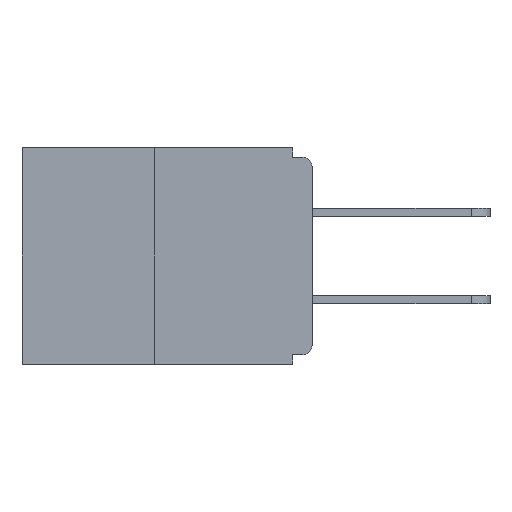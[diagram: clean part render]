
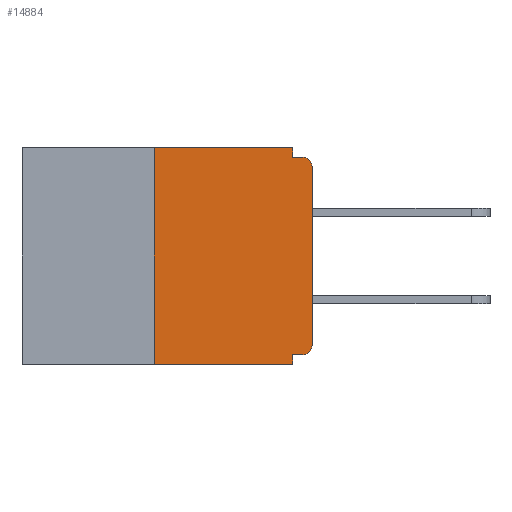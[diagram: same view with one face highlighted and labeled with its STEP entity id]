
A CAD part, left-side view. The second image highlights one B-rep face of the part: STEP entity #14884.
In plain terms, the highlighted planar face has unit normal (-1, 0, 0).
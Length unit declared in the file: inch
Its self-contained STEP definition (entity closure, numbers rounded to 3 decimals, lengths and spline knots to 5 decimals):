
#120 = ORIENTED_EDGE ( 'NONE', *, *, #15471, .T. ) ;
#579 = DIRECTION ( 'NONE',  ( 0., 0., -1. ) ) ;
#1184 = PLANE ( 'NONE',  #18767 ) ;
#1459 = CARTESIAN_POINT ( 'NONE',  ( 0., 0., 0. ) ) ;
#2770 = CARTESIAN_POINT ( 'NONE',  ( 0., 0.031, 0. ) ) ;
#2809 = VECTOR ( 'NONE', #9097, 39.37008 ) ;
#3345 = CARTESIAN_POINT ( 'NONE',  ( 0., 0.015, -0.328 ) ) ;
#3481 = VERTEX_POINT ( 'NONE', #20496 ) ;
#3826 = ORIENTED_EDGE ( 'NONE', *, *, #25433, .F. ) ;
#4639 = VERTEX_POINT ( 'NONE', #5701 ) ;
#4949 = ORIENTED_EDGE ( 'NONE', *, *, #5563, .T. ) ;
#4956 = VECTOR ( 'NONE', #579, 39.37008 ) ;
#5487 = EDGE_CURVE ( 'NONE', #21821, #3481, #13147, .T. ) ;
#5563 = EDGE_CURVE ( 'NONE', #14301, #21821, #7819, .T. ) ;
#5672 = ORIENTED_EDGE ( 'NONE', *, *, #7404, .F. ) ;
#5701 = CARTESIAN_POINT ( 'NONE',  ( 0., 0.031, 0. ) ) ;
#5748 = ORIENTED_EDGE ( 'NONE', *, *, #7896, .F. ) ;
#5768 = CARTESIAN_POINT ( 'NONE',  ( 0., 0.031, -0.328 ) ) ;
#5869 = VECTOR ( 'NONE', #22485, 39.37008 ) ;
#6130 = CARTESIAN_POINT ( 'NONE',  ( 0., 0., -0.328 ) ) ;
#6212 = AXIS2_PLACEMENT_3D ( 'NONE', #11804, #11997, #25696 ) ;
#6424 = EDGE_LOOP ( 'NONE', ( #20912, #5748, #14328, #3826, #5672, #4949, #8982, #120, #22084, #16648 ) ) ;
#6955 = AXIS2_PLACEMENT_3D ( 'NONE', #14535, #23785, #23608 ) ;
#7404 = EDGE_CURVE ( 'NONE', #14301, #9395, #20503, .T. ) ;
#7657 = CARTESIAN_POINT ( 'NONE',  ( 0., 0., -0.313 ) ) ;
#7669 = CIRCLE ( 'NONE', #6955, 0.015 ) ;
#7819 = CIRCLE ( 'NONE', #6212, 0.015 ) ;
#7896 = EDGE_CURVE ( 'NONE', #15224, #15062, #24730, .T. ) ;
#8139 = DIRECTION ( 'NONE',  ( 1., 0., 0. ) ) ;
#8410 = DIRECTION ( 'NONE',  ( 0., 1., 0. ) ) ;
#8478 = DIRECTION ( 'NONE',  ( 0., -1., 0. ) ) ;
#8982 = ORIENTED_EDGE ( 'NONE', *, *, #5487, .T. ) ;
#9097 = DIRECTION ( 'NONE',  ( 0., -1., 0. ) ) ;
#9395 = VERTEX_POINT ( 'NONE', #5768 ) ;
#9568 = LINE ( 'NONE', #15973, #2809 ) ;
#11019 = LINE ( 'NONE', #2770, #4956 ) ;
#11477 = CARTESIAN_POINT ( 'NONE',  ( 0., 0.031, -0.343 ) ) ;
#11804 = CARTESIAN_POINT ( 'NONE',  ( 0., 0.015, -0.313 ) ) ;
#11997 = DIRECTION ( 'NONE',  ( -1., 0., 0. ) ) ;
#12405 = CARTESIAN_POINT ( 'NONE',  ( 0., 0.015, -0.015 ) ) ;
#12442 = CARTESIAN_POINT ( 'NONE',  ( 0., 0.46, 0. ) ) ;
#12446 = EDGE_CURVE ( 'NONE', #4639, #26085, #11019, .T. ) ;
#13147 = LINE ( 'NONE', #1459, #27372 ) ;
#13225 = CARTESIAN_POINT ( 'NONE',  ( 0., 0.031, -0.343 ) ) ;
#13729 = VECTOR ( 'NONE', #8410, 39.37008 ) ;
#14010 = VECTOR ( 'NONE', #26837, 39.37008 ) ;
#14301 = VERTEX_POINT ( 'NONE', #3345 ) ;
#14328 = ORIENTED_EDGE ( 'NONE', *, *, #15155, .T. ) ;
#14535 = CARTESIAN_POINT ( 'NONE',  ( 0., 0.015, -0.03 ) ) ;
#14632 = DIRECTION ( 'NONE',  ( 0., 0., -1. ) ) ;
#14688 = CARTESIAN_POINT ( 'NONE',  ( 0., 0.031, -0.015 ) ) ;
#14884 = ADVANCED_FACE ( 'NONE', ( #25817 ), #1184, .F. ) ;
#15062 = VERTEX_POINT ( 'NONE', #26530 ) ;
#15155 = EDGE_CURVE ( 'NONE', #15224, #27470, #23383, .T. ) ;
#15190 = DIRECTION ( 'NONE',  ( 0., 0., 1. ) ) ;
#15224 = VERTEX_POINT ( 'NONE', #25034 ) ;
#15471 = EDGE_CURVE ( 'NONE', #3481, #19641, #7669, .T. ) ;
#15811 = CARTESIAN_POINT ( 'NONE',  ( 0., 0.46, -0.343 ) ) ;
#15973 = CARTESIAN_POINT ( 'NONE',  ( 0., 0.46, 0. ) ) ;
#16648 = ORIENTED_EDGE ( 'NONE', *, *, #12446, .F. ) ;
#17045 = CARTESIAN_POINT ( 'NONE',  ( 0., 0.25, 0. ) ) ;
#18767 = AXIS2_PLACEMENT_3D ( 'NONE', #12442, #8139, #14632 ) ;
#19641 = VERTEX_POINT ( 'NONE', #12405 ) ;
#20496 = CARTESIAN_POINT ( 'NONE',  ( 0., 0., -0.03 ) ) ;
#20503 = LINE ( 'NONE', #6130, #13729 ) ;
#20912 = ORIENTED_EDGE ( 'NONE', *, *, #22047, .F. ) ;
#21296 = DIRECTION ( 'NONE',  ( 0., 0., 1. ) ) ;
#21821 = VERTEX_POINT ( 'NONE', #7657 ) ;
#22047 = EDGE_CURVE ( 'NONE', #15062, #4639, #9568, .T. ) ;
#22084 = ORIENTED_EDGE ( 'NONE', *, *, #26910, .F. ) ;
#22124 = CARTESIAN_POINT ( 'NONE',  ( 0., 0., -0.015 ) ) ;
#22485 = DIRECTION ( 'NONE',  ( 0., -1., 0. ) ) ;
#23383 = LINE ( 'NONE', #15811, #5869 ) ;
#23608 = DIRECTION ( 'NONE',  ( 0., 0., -1. ) ) ;
#23698 = VECTOR ( 'NONE', #21296, 39.37008 ) ;
#23785 = DIRECTION ( 'NONE',  ( -1., 0., 0. ) ) ;
#23869 = LINE ( 'NONE', #22124, #25283 ) ;
#23950 = LINE ( 'NONE', #13225, #14010 ) ;
#24730 = LINE ( 'NONE', #17045, #23698 ) ;
#25034 = CARTESIAN_POINT ( 'NONE',  ( 0., 0.25, -0.343 ) ) ;
#25283 = VECTOR ( 'NONE', #8478, 39.37008 ) ;
#25433 = EDGE_CURVE ( 'NONE', #9395, #27470, #23950, .T. ) ;
#25696 = DIRECTION ( 'NONE',  ( 0., 0., -1. ) ) ;
#25817 = FACE_OUTER_BOUND ( 'NONE', #6424, .T. ) ;
#26085 = VERTEX_POINT ( 'NONE', #14688 ) ;
#26530 = CARTESIAN_POINT ( 'NONE',  ( 0., 0.25, 0. ) ) ;
#26837 = DIRECTION ( 'NONE',  ( 0., 0., -1. ) ) ;
#26910 = EDGE_CURVE ( 'NONE', #26085, #19641, #23869, .T. ) ;
#27372 = VECTOR ( 'NONE', #15190, 39.37008 ) ;
#27470 = VERTEX_POINT ( 'NONE', #11477 ) ;
